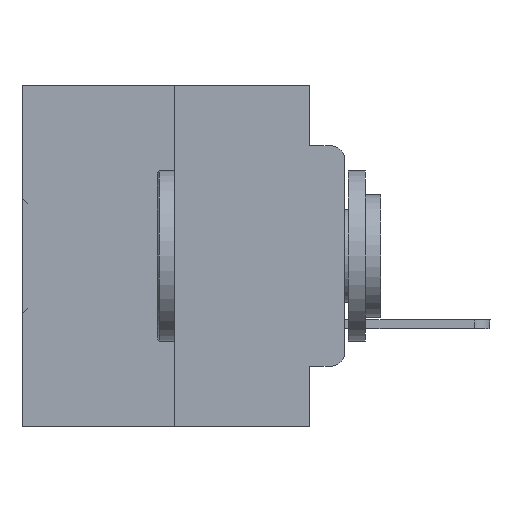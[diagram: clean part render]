
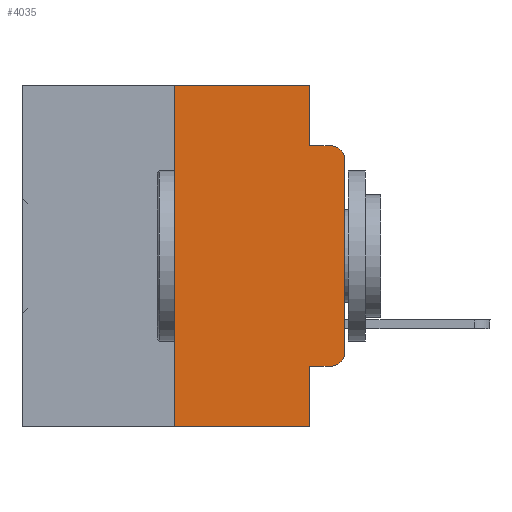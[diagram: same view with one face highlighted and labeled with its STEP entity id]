
A CAD part, left-side view. The second image highlights one B-rep face of the part: STEP entity #4035.
In plain terms, the highlighted planar face has unit normal (-1, 0, 0).
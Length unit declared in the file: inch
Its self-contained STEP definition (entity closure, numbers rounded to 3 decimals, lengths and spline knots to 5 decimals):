
#712 = VERTEX_POINT ( 'NONE', #26583 ) ;
#992 = LINE ( 'NONE', #14201, #26720 ) ;
#1019 = CARTESIAN_POINT ( 'NONE',  ( 0., 0.473, 0. ) ) ;
#1191 = VECTOR ( 'NONE', #10847, 39.37008 ) ;
#1208 = EDGE_CURVE ( 'NONE', #20221, #21423, #20790, .T. ) ;
#1321 = LINE ( 'NONE', #33897, #6203 ) ;
#1814 = ORIENTED_EDGE ( 'NONE', *, *, #18894, .F. ) ;
#2385 = EDGE_CURVE ( 'NONE', #11698, #20221, #24241, .T. ) ;
#2793 = ORIENTED_EDGE ( 'NONE', *, *, #6100, .T. ) ;
#3283 = EDGE_CURVE ( 'NONE', #24232, #12635, #14273, .T. ) ;
#3826 = ORIENTED_EDGE ( 'NONE', *, *, #2385, .T. ) ;
#4035 = ADVANCED_FACE ( 'NONE', ( #17719 ), #22850, .F. ) ;
#4195 = LINE ( 'NONE', #25517, #19931 ) ;
#4952 = DIRECTION ( 'NONE',  ( 0., -1., 0. ) ) ;
#5504 = ORIENTED_EDGE ( 'NONE', *, *, #20398, .T. ) ;
#5809 = CARTESIAN_POINT ( 'NONE',  ( 0., 0.25, 0. ) ) ;
#6022 = ORIENTED_EDGE ( 'NONE', *, *, #6968, .F. ) ;
#6100 = EDGE_CURVE ( 'NONE', #712, #27212, #19094, .T. ) ;
#6203 = VECTOR ( 'NONE', #14527, 39.37008 ) ;
#6968 = EDGE_CURVE ( 'NONE', #12635, #21545, #992, .T. ) ;
#7306 = CARTESIAN_POINT ( 'NONE',  ( 0., 0.25, -0.5 ) ) ;
#8051 = ORIENTED_EDGE ( 'NONE', *, *, #8831, .F. ) ;
#8116 = EDGE_LOOP ( 'NONE', ( #3826, #29555, #26094, #1814, #6022, #18714, #5504, #8051, #2793, #17190 ) ) ;
#8831 = EDGE_CURVE ( 'NONE', #712, #10003, #1321, .T. ) ;
#10003 = VERTEX_POINT ( 'NONE', #26157 ) ;
#10847 = DIRECTION ( 'NONE',  ( 0., 0., 1. ) ) ;
#11698 = VERTEX_POINT ( 'NONE', #30723 ) ;
#12123 = VECTOR ( 'NONE', #29504, 39.37008 ) ;
#12635 = VERTEX_POINT ( 'NONE', #32294 ) ;
#12787 = CARTESIAN_POINT ( 'NONE',  ( 0., 0.02, -0.4115 ) ) ;
#13227 = LINE ( 'NONE', #34018, #18564 ) ;
#13502 = AXIS2_PLACEMENT_3D ( 'NONE', #18907, #26008, #17711 ) ;
#14201 = CARTESIAN_POINT ( 'NONE',  ( 0., 0.473, 0. ) ) ;
#14273 = LINE ( 'NONE', #5809, #16322 ) ;
#14284 = EDGE_CURVE ( 'NONE', #23780, #21423, #13227, .T. ) ;
#14302 = CARTESIAN_POINT ( 'NONE',  ( 0., 0.051, 0. ) ) ;
#14527 = DIRECTION ( 'NONE',  ( 0., 0., -1. ) ) ;
#14580 = DIRECTION ( 'NONE',  ( 0., 0., -1. ) ) ;
#16322 = VECTOR ( 'NONE', #29973, 39.37008 ) ;
#17190 = ORIENTED_EDGE ( 'NONE', *, *, #25991, .T. ) ;
#17546 = DIRECTION ( 'NONE',  ( 1., 0., 0. ) ) ;
#17711 = DIRECTION ( 'NONE',  ( 0., 0., -1. ) ) ;
#17719 = FACE_OUTER_BOUND ( 'NONE', #8116, .T. ) ;
#18564 = VECTOR ( 'NONE', #4952, 39.37008 ) ;
#18714 = ORIENTED_EDGE ( 'NONE', *, *, #3283, .F. ) ;
#18894 = EDGE_CURVE ( 'NONE', #21545, #23780, #4195, .T. ) ;
#18907 = CARTESIAN_POINT ( 'NONE',  ( 0., 0.02, -0.3915 ) ) ;
#18951 = CARTESIAN_POINT ( 'NONE',  ( 0., 0., 0. ) ) ;
#19094 = LINE ( 'NONE', #21569, #12123 ) ;
#19420 = DIRECTION ( 'NONE',  ( 0., -1., 0. ) ) ;
#19668 = DIRECTION ( 'NONE',  ( 0., -1., 0. ) ) ;
#19931 = VECTOR ( 'NONE', #14580, 39.37008 ) ;
#20037 = DIRECTION ( 'NONE',  ( 0., 0., -1. ) ) ;
#20221 = VERTEX_POINT ( 'NONE', #22401 ) ;
#20240 = CIRCLE ( 'NONE', #13502, 0.02 ) ;
#20241 = AXIS2_PLACEMENT_3D ( 'NONE', #22459, #24582, #22628 ) ;
#20398 = EDGE_CURVE ( 'NONE', #24232, #10003, #26665, .T. ) ;
#20790 = CIRCLE ( 'NONE', #20241, 0.02 ) ;
#20943 = AXIS2_PLACEMENT_3D ( 'NONE', #1019, #17546, #20037 ) ;
#21423 = VERTEX_POINT ( 'NONE', #32467 ) ;
#21545 = VERTEX_POINT ( 'NONE', #14302 ) ;
#21569 = CARTESIAN_POINT ( 'NONE',  ( 0., 0.051, -0.4115 ) ) ;
#22401 = CARTESIAN_POINT ( 'NONE',  ( 0., 0., -0.1085 ) ) ;
#22459 = CARTESIAN_POINT ( 'NONE',  ( 0., 0.02, -0.1085 ) ) ;
#22628 = DIRECTION ( 'NONE',  ( 0., 0., -1. ) ) ;
#22850 = PLANE ( 'NONE',  #20943 ) ;
#23780 = VERTEX_POINT ( 'NONE', #31648 ) ;
#24232 = VERTEX_POINT ( 'NONE', #7306 ) ;
#24241 = LINE ( 'NONE', #18951, #1191 ) ;
#24582 = DIRECTION ( 'NONE',  ( -1., 0., 0. ) ) ;
#25517 = CARTESIAN_POINT ( 'NONE',  ( 0., 0.051, 0. ) ) ;
#25991 = EDGE_CURVE ( 'NONE', #27212, #11698, #20240, .T. ) ;
#26008 = DIRECTION ( 'NONE',  ( -1., 0., 0. ) ) ;
#26094 = ORIENTED_EDGE ( 'NONE', *, *, #14284, .F. ) ;
#26157 = CARTESIAN_POINT ( 'NONE',  ( 0., 0.051, -0.5 ) ) ;
#26583 = CARTESIAN_POINT ( 'NONE',  ( 0., 0.051, -0.4115 ) ) ;
#26665 = LINE ( 'NONE', #32805, #26797 ) ;
#26720 = VECTOR ( 'NONE', #19668, 39.37008 ) ;
#26797 = VECTOR ( 'NONE', #19420, 39.37008 ) ;
#27212 = VERTEX_POINT ( 'NONE', #12787 ) ;
#29504 = DIRECTION ( 'NONE',  ( 0., -1., 0. ) ) ;
#29555 = ORIENTED_EDGE ( 'NONE', *, *, #1208, .T. ) ;
#29973 = DIRECTION ( 'NONE',  ( 0., 0., 1. ) ) ;
#30723 = CARTESIAN_POINT ( 'NONE',  ( 0., 0., -0.3915 ) ) ;
#31648 = CARTESIAN_POINT ( 'NONE',  ( 0., 0.051, -0.0885 ) ) ;
#32294 = CARTESIAN_POINT ( 'NONE',  ( 0., 0.25, 0. ) ) ;
#32467 = CARTESIAN_POINT ( 'NONE',  ( 0., 0.02, -0.0885 ) ) ;
#32805 = CARTESIAN_POINT ( 'NONE',  ( 0., 0.473, -0.5 ) ) ;
#33897 = CARTESIAN_POINT ( 'NONE',  ( 0., 0.051, 0. ) ) ;
#34018 = CARTESIAN_POINT ( 'NONE',  ( 0., 0.051, -0.0885 ) ) ;
